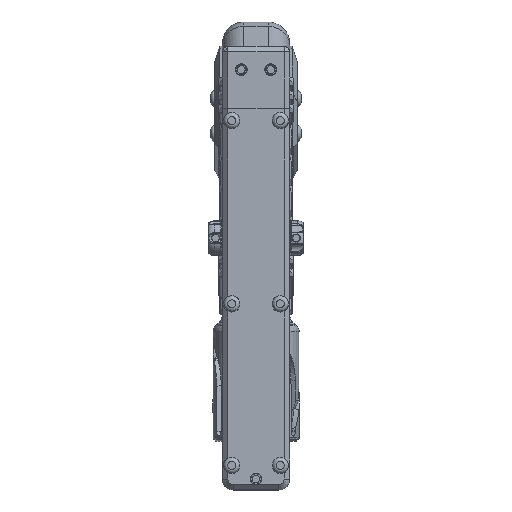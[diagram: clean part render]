
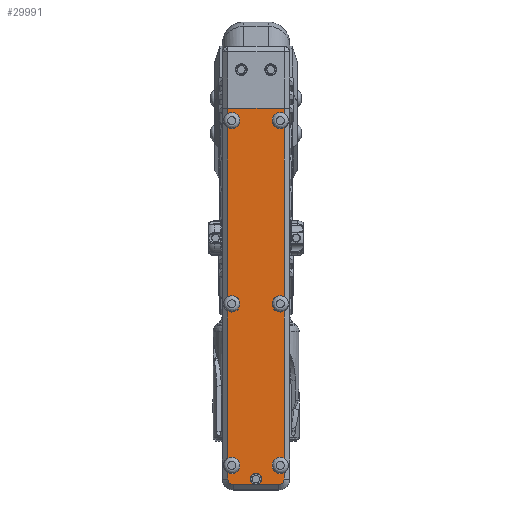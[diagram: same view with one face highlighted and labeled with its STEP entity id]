
A CAD part, top view. The second image highlights one B-rep face of the part: STEP entity #29991.
In plain terms, the highlighted planar face has unit normal (0, 0, 1).
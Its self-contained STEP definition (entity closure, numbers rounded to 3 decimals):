
#2474=FACE_BOUND($,#5620,.T.);
#2897=PLANE($,#32165);
#3709=FACE_OUTER_BOUND($,#5619,.T.);
#5619=EDGE_LOOP($,(#20985,#20986,#20987,#20988,#20989,#20990,#20991,#20992,
#20993,#20994,#20995,#20996,#20997,#20998,#20999,#21000,#21001,#21002));
#5620=EDGE_LOOP($,(#21003));
#7855=LINE($,#43734,#9554);
#7857=LINE($,#43742,#9556);
#7861=LINE($,#43750,#9560);
#7863=LINE($,#43758,#9562);
#7867=LINE($,#43772,#9566);
#7870=LINE($,#43783,#9569);
#7873=LINE($,#43789,#9572);
#7875=LINE($,#43797,#9574);
#7876=LINE($,#43802,#9575);
#7877=LINE($,#43815,#9576);
#9554=VECTOR($,#35644,6.269);
#9556=VECTOR($,#35650,0.195);
#9560=VECTOR($,#35654,0.239);
#9562=VECTOR($,#35660,5.469);
#9566=VECTOR($,#35674,1.7);
#9569=VECTOR($,#35687,0.239);
#9572=VECTOR($,#35690,0.195);
#9574=VECTOR($,#35696,6.269);
#9575=VECTOR($,#35701,5.469);
#9576=VECTOR($,#35726,2.1);
#11208=CIRCLE($,#32140,0.2);
#11210=CIRCLE($,#32144,0.2);
#11213=CIRCLE($,#32155,0.305);
#11215=CIRCLE($,#32158,0.305);
#11216=CIRCLE($,#32160,0.305);
#11217=CIRCLE($,#32162,0.305);
#11218=CIRCLE($,#32166,0.305);
#11219=CIRCLE($,#32167,0.305);
#11220=CIRCLE($,#32168,0.14);
#12610=VERTEX_POINT($,#43731);
#12611=VERTEX_POINT($,#43733);
#12614=VERTEX_POINT($,#43739);
#12615=VERTEX_POINT($,#43741);
#12618=VERTEX_POINT($,#43747);
#12619=VERTEX_POINT($,#43749);
#12622=VERTEX_POINT($,#43755);
#12623=VERTEX_POINT($,#43757);
#12626=VERTEX_POINT($,#43764);
#12628=VERTEX_POINT($,#43770);
#12630=VERTEX_POINT($,#43776);
#12631=VERTEX_POINT($,#43781);
#12633=VERTEX_POINT($,#43786);
#12634=VERTEX_POINT($,#43788);
#12637=VERTEX_POINT($,#43794);
#12638=VERTEX_POINT($,#43796);
#12639=VERTEX_POINT($,#43799);
#12640=VERTEX_POINT($,#43801);
#12649=VERTEX_POINT($,#43838);
#15825=EDGE_CURVE($,#12610,#12611,#7855,.T.);
#15829=EDGE_CURVE($,#12614,#12615,#7857,.T.);
#15833=EDGE_CURVE($,#12618,#12619,#7861,.T.);
#15837=EDGE_CURVE($,#12622,#12623,#7863,.T.);
#15841=EDGE_CURVE($,#12626,#12618,#11208,.T.);
#15844=EDGE_CURVE($,#12628,#12626,#7867,.T.);
#15847=EDGE_CURVE($,#12630,#12628,#11210,.T.);
#15850=EDGE_CURVE($,#12631,#12630,#7870,.T.);
#15853=EDGE_CURVE($,#12633,#12634,#7873,.T.);
#15857=EDGE_CURVE($,#12637,#12638,#7875,.T.);
#15860=EDGE_CURVE($,#12639,#12640,#7876,.T.);
#15863=EDGE_CURVE($,#12610,#12623,#11213,.T.);
#15865=EDGE_CURVE($,#12622,#12619,#11215,.T.);
#15866=EDGE_CURVE($,#12631,#12640,#11216,.T.);
#15867=EDGE_CURVE($,#12639,#12638,#11217,.T.);
#15868=EDGE_CURVE($,#12633,#12615,#7877,.T.);
#15879=EDGE_CURVE($,#12637,#12634,#11218,.T.);
#15880=EDGE_CURVE($,#12614,#12611,#11219,.T.);
#15881=EDGE_CURVE($,#12649,#12649,#11220,.F.);
#20985=ORIENTED_EDGE($,*,*,#15825,.F.);
#20986=ORIENTED_EDGE($,*,*,#15863,.T.);
#20987=ORIENTED_EDGE($,*,*,#15837,.F.);
#20988=ORIENTED_EDGE($,*,*,#15865,.T.);
#20989=ORIENTED_EDGE($,*,*,#15833,.F.);
#20990=ORIENTED_EDGE($,*,*,#15841,.F.);
#20991=ORIENTED_EDGE($,*,*,#15844,.F.);
#20992=ORIENTED_EDGE($,*,*,#15847,.F.);
#20993=ORIENTED_EDGE($,*,*,#15850,.F.);
#20994=ORIENTED_EDGE($,*,*,#15866,.T.);
#20995=ORIENTED_EDGE($,*,*,#15860,.F.);
#20996=ORIENTED_EDGE($,*,*,#15867,.T.);
#20997=ORIENTED_EDGE($,*,*,#15857,.F.);
#20998=ORIENTED_EDGE($,*,*,#15879,.T.);
#20999=ORIENTED_EDGE($,*,*,#15853,.F.);
#21000=ORIENTED_EDGE($,*,*,#15868,.T.);
#21001=ORIENTED_EDGE($,*,*,#15829,.F.);
#21002=ORIENTED_EDGE($,*,*,#15880,.T.);
#21003=ORIENTED_EDGE($,*,*,#15881,.T.);
#29991=ADVANCED_FACE($,(#3709,#2474),#2897,.T.);
#32140=AXIS2_PLACEMENT_3D($,#43766,#35667,#35668);
#32144=AXIS2_PLACEMENT_3D($,#43778,#35679,#35680);
#32155=AXIS2_PLACEMENT_3D($,#43806,#35708,#35709);
#32158=AXIS2_PLACEMENT_3D($,#43809,#35714,#35715);
#32160=AXIS2_PLACEMENT_3D($,#43811,#35718,#35719);
#32162=AXIS2_PLACEMENT_3D($,#43813,#35722,#35723);
#32165=AXIS2_PLACEMENT_3D($,#43835,#35739,#35740);
#32166=AXIS2_PLACEMENT_3D($,#43836,#35741,#35742);
#32167=AXIS2_PLACEMENT_3D($,#43837,#35743,#35744);
#32168=AXIS2_PLACEMENT_3D($,#43839,#35745,#35746);
#35644=DIRECTION($,(0.,1.,0.));
#35650=DIRECTION($,(0.,1.,0.));
#35654=DIRECTION($,(0.,1.,0.));
#35660=DIRECTION($,(0.,1.,0.));
#35667=DIRECTION('center_axis',(0.,0.,-1.));
#35668=DIRECTION('ref_axis',(-0.707,-0.707,0.));
#35674=DIRECTION($,(-1.,0.,0.));
#35679=DIRECTION('center_axis',(0.,0.,-1.));
#35680=DIRECTION('ref_axis',(0.707,-0.707,0.));
#35687=DIRECTION($,(0.,-1.,0.));
#35690=DIRECTION($,(0.,-1.,0.));
#35696=DIRECTION($,(0.,-1.,0.));
#35701=DIRECTION($,(0.,-1.,0.));
#35708=DIRECTION('center_axis',(0.,0.,-1.));
#35709=DIRECTION('ref_axis',(-1.,0.,0.));
#35714=DIRECTION('center_axis',(0.,0.,-1.));
#35715=DIRECTION('ref_axis',(-1.,0.,0.));
#35718=DIRECTION('center_axis',(0.,0.,-1.));
#35719=DIRECTION('ref_axis',(-1.,0.,0.));
#35722=DIRECTION('center_axis',(0.,0.,-1.));
#35723=DIRECTION('ref_axis',(-1.,0.,0.));
#35726=DIRECTION($,(-1.,0.,0.));
#35739=DIRECTION('center_axis',(0.,0.,1.));
#35740=DIRECTION('ref_axis',(-1.,0.,0.));
#35741=DIRECTION('center_axis',(0.,0.,-1.));
#35742=DIRECTION('ref_axis',(-1.,0.,0.));
#35743=DIRECTION('center_axis',(0.,0.,-1.));
#35744=DIRECTION('ref_axis',(-1.,0.,0.));
#35745=DIRECTION('center_axis',(0.,0.,1.));
#35746=DIRECTION('ref_axis',(0.,-1.,0.));
#43731=CARTESIAN_POINT('',(-9.497,10.199,12.378));
#43733=CARTESIAN_POINT('',(-9.497,16.468,12.378));
#43734=CARTESIAN_POINT($,(-9.497,18.822,12.378));
#43739=CARTESIAN_POINT('',(-9.497,16.999,12.378));
#43741=CARTESIAN_POINT('',(-9.497,17.194,12.378));
#43742=CARTESIAN_POINT($,(-9.497,18.822,12.378));
#43747=CARTESIAN_POINT('',(-9.497,3.429,12.378));
#43749=CARTESIAN_POINT('',(-9.497,3.668,12.378));
#43750=CARTESIAN_POINT($,(-9.497,18.822,12.378));
#43755=CARTESIAN_POINT('',(-9.497,4.199,12.378));
#43757=CARTESIAN_POINT('',(-9.497,9.668,12.378));
#43758=CARTESIAN_POINT($,(-9.497,18.822,12.378));
#43764=CARTESIAN_POINT('',(-9.297,3.229,12.378));
#43766=CARTESIAN_POINT('Origin',(-9.297,3.429,12.378));
#43770=CARTESIAN_POINT('',(-7.597,3.229,12.378));
#43772=CARTESIAN_POINT($,(-8.239,3.229,12.378));
#43776=CARTESIAN_POINT('',(-7.397,3.429,12.378));
#43778=CARTESIAN_POINT('Origin',(-7.597,3.429,12.378));
#43781=CARTESIAN_POINT('',(-7.397,3.668,12.378));
#43783=CARTESIAN_POINT($,(-7.397,10.889,12.378));
#43786=CARTESIAN_POINT('',(-7.397,17.194,12.378));
#43788=CARTESIAN_POINT('',(-7.397,16.999,12.378));
#43789=CARTESIAN_POINT($,(-7.397,10.889,12.378));
#43794=CARTESIAN_POINT('',(-7.397,16.468,12.378));
#43796=CARTESIAN_POINT('',(-7.397,10.199,12.378));
#43797=CARTESIAN_POINT($,(-7.397,10.889,12.378));
#43799=CARTESIAN_POINT('',(-7.397,9.668,12.378));
#43801=CARTESIAN_POINT('',(-7.397,4.199,12.378));
#43802=CARTESIAN_POINT($,(-7.397,10.889,12.378));
#43806=CARTESIAN_POINT('Origin',(-9.347,9.934,12.378));
#43809=CARTESIAN_POINT('Origin',(-9.347,3.934,12.378));
#43811=CARTESIAN_POINT('Origin',(-7.547,3.934,12.378));
#43813=CARTESIAN_POINT('Origin',(-7.547,9.934,12.378));
#43815=CARTESIAN_POINT($,(-7.814,17.194,12.378));
#43835=CARTESIAN_POINT('Origin',(-7.18,18.35,12.378));
#43836=CARTESIAN_POINT('Origin',(-7.547,16.734,12.378));
#43837=CARTESIAN_POINT('Origin',(-9.347,16.734,12.378));
#43838=CARTESIAN_POINT('',(-8.447,3.569,12.378));
#43839=CARTESIAN_POINT('Origin',(-8.447,3.429,12.378));
